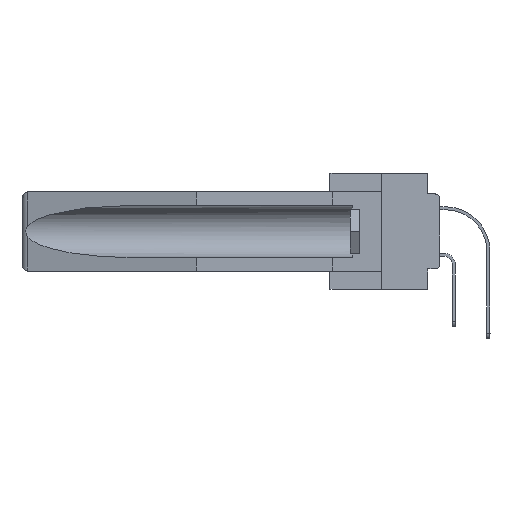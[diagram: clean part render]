
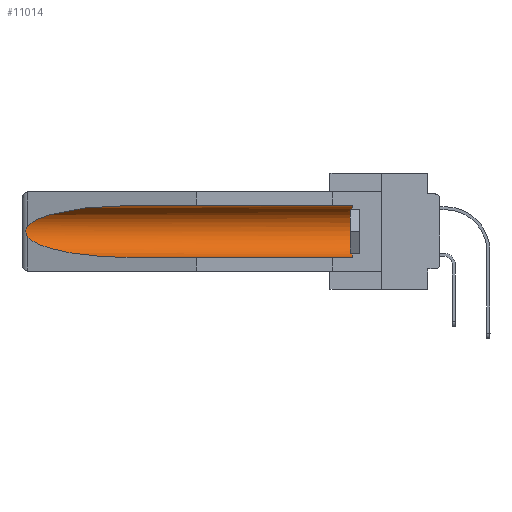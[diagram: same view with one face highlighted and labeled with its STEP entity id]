
A CAD part, left-side view. The second image highlights one B-rep face of the part: STEP entity #11014.
In plain terms, the highlighted cylindrical face has radius 2.857 mm (diameter 5.715 mm), a partial arc.
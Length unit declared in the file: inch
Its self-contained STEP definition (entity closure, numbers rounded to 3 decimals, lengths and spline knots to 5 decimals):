
#290 = CARTESIAN_POINT ( 'NONE',  ( 0.155, 0.126, -0.059 ) ) ;
#695 = ORIENTED_EDGE ( 'NONE', *, *, #37595, .T. ) ;
#2122 = CYLINDRICAL_SURFACE ( 'NONE', #15152, 0.1125 ) ;
#2901 = LINE ( 'NONE', #11986, #4012 ) ;
#3125 = CARTESIAN_POINT ( 'NONE',  ( 0.21114, 1.30732, -0.059 ) ) ;
#3930 = CARTESIAN_POINT ( 'NONE',  ( 0.26537, 1.52718, -0.19328 ) ) ;
#4007 = EDGE_LOOP ( 'NONE', ( #18667, #695, #6746, #38116, #4896, #20807 ) ) ;
#4012 = VECTOR ( 'NONE', #8506, 39.37008 ) ;
#4896 = ORIENTED_EDGE ( 'NONE', *, *, #29297, .T. ) ;
#5032 = DIRECTION ( 'NONE',  ( 0., 1., 0. ) ) ;
#5416 = VERTEX_POINT ( 'NONE', #14308 ) ;
#5549 =( BOUNDED_CURVE ( )  B_SPLINE_CURVE ( 3, ( #17813, #3125, #20931, #22231 ),
 .UNSPECIFIED., .F., .F. ) 
 B_SPLINE_CURVE_WITH_KNOTS ( ( 4, 4 ),
 ( 4.71239, 6.08839 ),
 .UNSPECIFIED. ) 
 CURVE ( )  GEOMETRIC_REPRESENTATION_ITEM ( )  RATIONAL_B_SPLINE_CURVE ( ( 1., 0.848, 0.848, 1. ) ) 
 REPRESENTATION_ITEM ( '' )  );
#5611 = LINE ( 'NONE', #17583, #22257 ) ;
#5978 = VERTEX_POINT ( 'NONE', #290 ) ;
#6746 = ORIENTED_EDGE ( 'NONE', *, *, #24713, .T. ) ;
#7377 = CARTESIAN_POINT ( 'NONE',  ( 0.21114, 1.30732, -0.284 ) ) ;
#8506 = DIRECTION ( 'NONE',  ( 0., 1., 0. ) ) ;
#8625 = VERTEX_POINT ( 'NONE', #13092 ) ;
#11014 = ADVANCED_FACE ( 'NONE', ( #28630 ), #2122, .F. ) ;
#11591 = VERTEX_POINT ( 'NONE', #35138 ) ;
#11986 = CARTESIAN_POINT ( 'NONE',  ( 0.155, -0.30754, -0.284 ) ) ;
#12034 = CARTESIAN_POINT ( 'NONE',  ( 0.155, 0.126, -0.1715 ) ) ;
#13000 = CARTESIAN_POINT ( 'NONE',  ( 0.2673, 1.53269, -0.17917 ) ) ;
#13092 = CARTESIAN_POINT ( 'NONE',  ( 0.155, 0.126, -0.284 ) ) ;
#13202 = CARTESIAN_POINT ( 'NONE',  ( 0.2675, 1.53308, -0.16763 ) ) ;
#13910 = DIRECTION ( 'NONE',  ( 0., 0., 1. ) ) ;
#14308 = CARTESIAN_POINT ( 'NONE',  ( 0.26537, 1.52718, -0.19328 ) ) ;
#14731 = DIRECTION ( 'NONE',  ( 0., 0., 1. ) ) ;
#15152 = AXIS2_PLACEMENT_3D ( 'NONE', #21944, #5032, #13910 ) ;
#15406 = EDGE_CURVE ( 'NONE', #8625, #29290, #2901, .T. ) ;
#17199 = DIRECTION ( 'NONE',  ( 0., 1., 0. ) ) ;
#17583 = CARTESIAN_POINT ( 'NONE',  ( 0.155, -0.30754, -0.059 ) ) ;
#17813 = CARTESIAN_POINT ( 'NONE',  ( 0.155, 1.07973, -0.059 ) ) ;
#18667 = ORIENTED_EDGE ( 'NONE', *, *, #28059, .T. ) ;
#19917 = B_SPLINE_CURVE_WITH_KNOTS ( 'NONE', 3,
 ( #25594, #36992, #33912, #25404, #13202, #37175, #13000, #31208, #27724, #33733 ),
 .UNSPECIFIED., .F., .F.,
 ( 4, 2, 2, 2, 4 ),
 ( 0., 0.00029, 0.00058, 0.00087, 0.00117 ),
 .UNSPECIFIED. ) ;
#20807 = ORIENTED_EDGE ( 'NONE', *, *, #21946, .T. ) ;
#20931 = CARTESIAN_POINT ( 'NONE',  ( 0.25451, 1.48313, -0.09465 ) ) ;
#21743 = CARTESIAN_POINT ( 'NONE',  ( 0.155, 1.07973, -0.284 ) ) ;
#21944 = CARTESIAN_POINT ( 'NONE',  ( 0.155, -0.30754, -0.1715 ) ) ;
#21946 = EDGE_CURVE ( 'NONE', #5978, #11591, #5611, .T. ) ;
#22231 = CARTESIAN_POINT ( 'NONE',  ( 0.26537, 1.52718, -0.14972 ) ) ;
#22257 = VECTOR ( 'NONE', #17199, 39.37008 ) ;
#24713 = EDGE_CURVE ( 'NONE', #5416, #29290, #26575, .T. ) ;
#25404 = CARTESIAN_POINT ( 'NONE',  ( 0.2673, 1.5327, -0.16383 ) ) ;
#25594 = CARTESIAN_POINT ( 'NONE',  ( 0.26537, 1.52718, -0.14972 ) ) ;
#26575 =( BOUNDED_CURVE ( )  B_SPLINE_CURVE ( 3, ( #3930, #30431, #7377, #21743 ),
 .UNSPECIFIED., .F., .F. ) 
 B_SPLINE_CURVE_WITH_KNOTS ( ( 4, 4 ),
 ( 0.1948, 1.5708 ),
 .UNSPECIFIED. ) 
 CURVE ( )  GEOMETRIC_REPRESENTATION_ITEM ( )  RATIONAL_B_SPLINE_CURVE ( ( 1., 0.848, 0.848, 1. ) ) 
 REPRESENTATION_ITEM ( '' )  );
#27139 = CARTESIAN_POINT ( 'NONE',  ( 0.155, 1.07973, -0.284 ) ) ;
#27724 = CARTESIAN_POINT ( 'NONE',  ( 0.26597, 1.5296, -0.19026 ) ) ;
#28059 = EDGE_CURVE ( 'NONE', #11591, #32491, #5549, .T. ) ;
#28129 = AXIS2_PLACEMENT_3D ( 'NONE', #12034, #32556, #14731 ) ;
#28630 = FACE_OUTER_BOUND ( 'NONE', #4007, .T. ) ;
#29290 = VERTEX_POINT ( 'NONE', #27139 ) ;
#29297 = EDGE_CURVE ( 'NONE', #8625, #5978, #33690, .T. ) ;
#30431 = CARTESIAN_POINT ( 'NONE',  ( 0.25451, 1.48313, -0.24835 ) ) ;
#31208 = CARTESIAN_POINT ( 'NONE',  ( 0.26655, 1.53094, -0.18657 ) ) ;
#32491 = VERTEX_POINT ( 'NONE', #37261 ) ;
#32556 = DIRECTION ( 'NONE',  ( 0., -1., 0. ) ) ;
#33690 = CIRCLE ( 'NONE', #28129, 0.1125 ) ;
#33733 = CARTESIAN_POINT ( 'NONE',  ( 0.26537, 1.52718, -0.19328 ) ) ;
#33912 = CARTESIAN_POINT ( 'NONE',  ( 0.26654, 1.53092, -0.15636 ) ) ;
#35138 = CARTESIAN_POINT ( 'NONE',  ( 0.155, 1.07973, -0.059 ) ) ;
#36992 = CARTESIAN_POINT ( 'NONE',  ( 0.26597, 1.52961, -0.15275 ) ) ;
#37175 = CARTESIAN_POINT ( 'NONE',  ( 0.2675, 1.53308, -0.17534 ) ) ;
#37261 = CARTESIAN_POINT ( 'NONE',  ( 0.26537, 1.52718, -0.14972 ) ) ;
#37595 = EDGE_CURVE ( 'NONE', #32491, #5416, #19917, .T. ) ;
#38116 = ORIENTED_EDGE ( 'NONE', *, *, #15406, .F. ) ;
